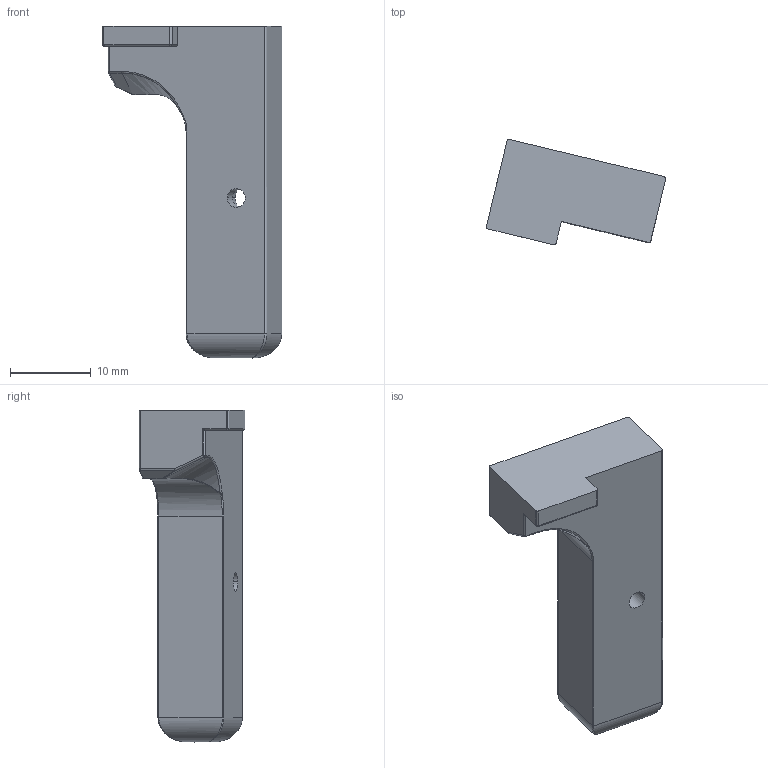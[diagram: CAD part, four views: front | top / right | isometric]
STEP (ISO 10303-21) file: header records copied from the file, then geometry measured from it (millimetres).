
FILE_DESCRIPTION (( 'STEP AP203' ), '1' );
FILE_NAME ('Mag Catch Compression Spring.STEP', ( '' ), ( '' ), 'SwSTEP 2.0', 'SolidWorks 2019', '' );
FILE_SCHEMA (( 'CONFIG_CONTROL_DESIGN' ));
Length unit declared in the file: millimetre
Products named in the file (1): Mag Catch Compression Spring
Bounding box: 22.15 x 13.04 x 41 mm (x, y, z)
Volume: 4114.7 mm3; surface area: 2079.5 mm2
Topology: 1 solids, 1 shells, 69 faces, 167 edges, 93 vertices
Faces by surface type: cylinder 33, plane 15, bspline 14, sphere 4, torus 3
Entity records: 2792 total; most frequent: CARTESIAN_POINT 1278, ORIENTED_EDGE 312, DIRECTION 269, EDGE_CURVE 156, AXIS2_PLACEMENT_3D 102, VERTEX_POINT 91, EDGE_LOOP 73, FACE_OUTER_BOUND 69
